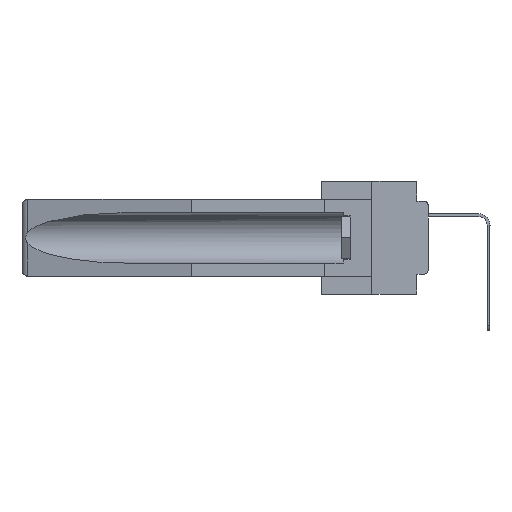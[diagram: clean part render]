
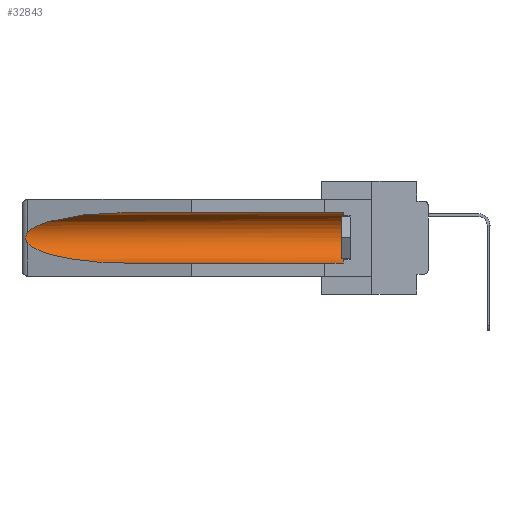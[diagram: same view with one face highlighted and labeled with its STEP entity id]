
A CAD part, left-side view. The second image highlights one B-rep face of the part: STEP entity #32843.
In plain terms, the highlighted cylindrical face has radius 2.857 mm (diameter 5.715 mm), a partial arc.
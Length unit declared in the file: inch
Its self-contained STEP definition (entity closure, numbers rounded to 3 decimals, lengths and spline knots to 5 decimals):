
#546 = CARTESIAN_POINT ( 'NONE',  ( 0.21114, 1.30732, -0.284 ) ) ;
#2089 = EDGE_CURVE ( 'NONE', #11181, #30196, #3308, .T. ) ;
#2269 = ORIENTED_EDGE ( 'NONE', *, *, #21244, .T. ) ;
#2913 = DIRECTION ( 'NONE',  ( 0., 0., 1. ) ) ;
#3308 = LINE ( 'NONE', #13082, #15145 ) ;
#4868 = B_SPLINE_CURVE_WITH_KNOTS ( 'NONE', 3,
 ( #10728, #22191, #13405, #36312, #27569, #24640, #19514, #36078, #19050, #5102 ),
 .UNSPECIFIED., .F., .F.,
 ( 4, 2, 2, 2, 4 ),
 ( 0., 0.00029, 0.00058, 0.00087, 0.00117 ),
 .UNSPECIFIED. ) ;
#5102 = CARTESIAN_POINT ( 'NONE',  ( 0.26537, 1.52718, -0.19328 ) ) ;
#5428 = CARTESIAN_POINT ( 'NONE',  ( 0.26537, 1.52718, -0.14972 ) ) ;
#5759 = DIRECTION ( 'NONE',  ( 0., 1., 0. ) ) ;
#6319 = CARTESIAN_POINT ( 'NONE',  ( 0.21114, 1.30732, -0.059 ) ) ;
#7178 = FACE_OUTER_BOUND ( 'NONE', #20844, .T. ) ;
#7317 = CARTESIAN_POINT ( 'NONE',  ( 0.155, 0.126, -0.059 ) ) ;
#10728 = CARTESIAN_POINT ( 'NONE',  ( 0.26537, 1.52718, -0.14972 ) ) ;
#11181 = VERTEX_POINT ( 'NONE', #34008 ) ;
#11253 = CARTESIAN_POINT ( 'NONE',  ( 0.155, -0.30754, -0.1715 ) ) ;
#11464 = DIRECTION ( 'NONE',  ( 0., 0., 1. ) ) ;
#11734 = ORIENTED_EDGE ( 'NONE', *, *, #20169, .T. ) ;
#13082 = CARTESIAN_POINT ( 'NONE',  ( 0.155, -0.30754, -0.284 ) ) ;
#13373 = DIRECTION ( 'NONE',  ( 0., 1., 0. ) ) ;
#13405 = CARTESIAN_POINT ( 'NONE',  ( 0.26654, 1.53092, -0.15636 ) ) ;
#14281 = ORIENTED_EDGE ( 'NONE', *, *, #31201, .T. ) ;
#14354 = VECTOR ( 'NONE', #13373, 39.37008 ) ;
#14615 = CARTESIAN_POINT ( 'NONE',  ( 0.26537, 1.52718, -0.14972 ) ) ;
#15145 = VECTOR ( 'NONE', #24434, 39.37008 ) ;
#16214 = CIRCLE ( 'NONE', #31613, 0.1125 ) ;
#17236 = CARTESIAN_POINT ( 'NONE',  ( 0.26537, 1.52718, -0.19328 ) ) ;
#17338 = CARTESIAN_POINT ( 'NONE',  ( 0.155, 0.126, -0.1715 ) ) ;
#17574 = VERTEX_POINT ( 'NONE', #5428 ) ;
#17731 = CARTESIAN_POINT ( 'NONE',  ( 0.155, 1.07973, -0.284 ) ) ;
#18051 = AXIS2_PLACEMENT_3D ( 'NONE', #11253, #5759, #2913 ) ;
#19050 = CARTESIAN_POINT ( 'NONE',  ( 0.26597, 1.5296, -0.19026 ) ) ;
#19071 = CARTESIAN_POINT ( 'NONE',  ( 0.155, 1.07973, -0.059 ) ) ;
#19514 = CARTESIAN_POINT ( 'NONE',  ( 0.2673, 1.53269, -0.17917 ) ) ;
#20030 = LINE ( 'NONE', #35694, #14354 ) ;
#20169 = EDGE_CURVE ( 'NONE', #11181, #28948, #16214, .T. ) ;
#20472 = CARTESIAN_POINT ( 'NONE',  ( 0.25451, 1.48313, -0.09465 ) ) ;
#20844 = EDGE_LOOP ( 'NONE', ( #27451, #21894, #14281, #21220, #11734, #2269 ) ) ;
#21220 = ORIENTED_EDGE ( 'NONE', *, *, #2089, .F. ) ;
#21244 = EDGE_CURVE ( 'NONE', #28948, #31468, #20030, .T. ) ;
#21894 = ORIENTED_EDGE ( 'NONE', *, *, #25974, .T. ) ;
#22191 = CARTESIAN_POINT ( 'NONE',  ( 0.26597, 1.52961, -0.15275 ) ) ;
#24425 = CARTESIAN_POINT ( 'NONE',  ( 0.155, 1.07973, -0.284 ) ) ;
#24434 = DIRECTION ( 'NONE',  ( 0., 1., 0. ) ) ;
#24640 = CARTESIAN_POINT ( 'NONE',  ( 0.2675, 1.53308, -0.17534 ) ) ;
#25974 = EDGE_CURVE ( 'NONE', #17574, #27421, #4868, .T. ) ;
#26187 = EDGE_CURVE ( 'NONE', #31468, #17574, #34691, .T. ) ;
#27421 = VERTEX_POINT ( 'NONE', #32016 ) ;
#27451 = ORIENTED_EDGE ( 'NONE', *, *, #26187, .T. ) ;
#27569 = CARTESIAN_POINT ( 'NONE',  ( 0.2675, 1.53308, -0.16763 ) ) ;
#28401 =( BOUNDED_CURVE ( )  B_SPLINE_CURVE ( 3, ( #17236, #31298, #546, #17731 ),
 .UNSPECIFIED., .F., .F. ) 
 B_SPLINE_CURVE_WITH_KNOTS ( ( 4, 4 ),
 ( 0.1948, 1.5708 ),
 .UNSPECIFIED. ) 
 CURVE ( )  GEOMETRIC_REPRESENTATION_ITEM ( )  RATIONAL_B_SPLINE_CURVE ( ( 1., 0.848, 0.848, 1. ) ) 
 REPRESENTATION_ITEM ( '' )  );
#28948 = VERTEX_POINT ( 'NONE', #7317 ) ;
#30196 = VERTEX_POINT ( 'NONE', #24425 ) ;
#30913 = DIRECTION ( 'NONE',  ( 0., -1., 0. ) ) ;
#31201 = EDGE_CURVE ( 'NONE', #27421, #30196, #28401, .T. ) ;
#31298 = CARTESIAN_POINT ( 'NONE',  ( 0.25451, 1.48313, -0.24835 ) ) ;
#31468 = VERTEX_POINT ( 'NONE', #19071 ) ;
#31613 = AXIS2_PLACEMENT_3D ( 'NONE', #17338, #30913, #11464 ) ;
#31624 = CARTESIAN_POINT ( 'NONE',  ( 0.155, 1.07973, -0.059 ) ) ;
#31722 = CYLINDRICAL_SURFACE ( 'NONE', #18051, 0.1125 ) ;
#32016 = CARTESIAN_POINT ( 'NONE',  ( 0.26537, 1.52718, -0.19328 ) ) ;
#32843 = ADVANCED_FACE ( 'NONE', ( #7178 ), #31722, .F. ) ;
#34008 = CARTESIAN_POINT ( 'NONE',  ( 0.155, 0.126, -0.284 ) ) ;
#34691 =( BOUNDED_CURVE ( )  B_SPLINE_CURVE ( 3, ( #31624, #6319, #20472, #14615 ),
 .UNSPECIFIED., .F., .F. ) 
 B_SPLINE_CURVE_WITH_KNOTS ( ( 4, 4 ),
 ( 4.71239, 6.08839 ),
 .UNSPECIFIED. ) 
 CURVE ( )  GEOMETRIC_REPRESENTATION_ITEM ( )  RATIONAL_B_SPLINE_CURVE ( ( 1., 0.848, 0.848, 1. ) ) 
 REPRESENTATION_ITEM ( '' )  );
#35694 = CARTESIAN_POINT ( 'NONE',  ( 0.155, -0.30754, -0.059 ) ) ;
#36078 = CARTESIAN_POINT ( 'NONE',  ( 0.26655, 1.53094, -0.18657 ) ) ;
#36312 = CARTESIAN_POINT ( 'NONE',  ( 0.2673, 1.5327, -0.16383 ) ) ;
